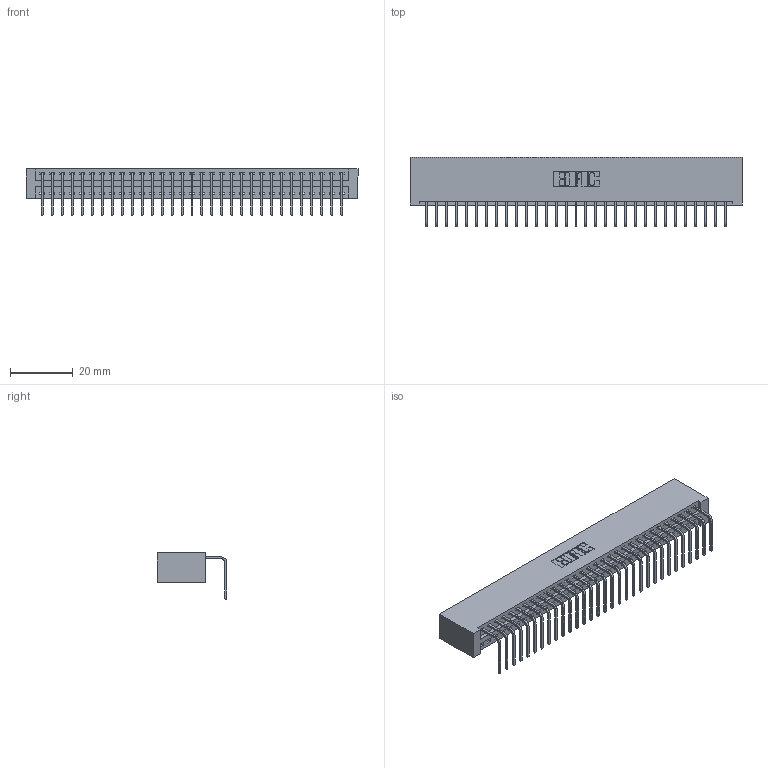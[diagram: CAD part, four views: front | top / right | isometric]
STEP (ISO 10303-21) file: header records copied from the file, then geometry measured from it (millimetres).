
FILE_DESCRIPTION (( 'STEP AP203' ), '1' );
FILE_NAME ('396-031-558-101.STEP', '2018-09-05T09:18:18', ( '' ), ( '' ), 'SwSTEP 2.0', 'SolidWorks 2016', '' );
FILE_SCHEMA (( 'CONFIG_CONTROL_DESIGN' ));
Length unit declared in the file: inch
Products named in the file (3): 346 Part_No Mounting Lugs; 345-292-001_558 Tail - 2; 396-031-558-101
Assembly tree (32 placements, depth 2):
  396-031-558-101
    346 Part_No Mounting Lugs
    345-292-001_558 Tail - 2  x31
Bounding box: 105.66 x 22.16 x 14.73 mm (x, y, z)
Volume: 10691.3 mm3; surface area: 13935.3 mm2
Topology: 32 solids, 32 shells, 1974 faces, 5947 edges, 3922 vertices
Faces by surface type: plane 1374, cylinder 600
Entity records: 20527 total; most frequent: CARTESIAN_POINT 3529, ORIENTED_EDGE 3494, DIRECTION 3121, EDGE_CURVE 1747, LINE 1499, VECTOR 1499, VERTEX_POINT 1162, AXIS2_PLACEMENT_3D 811
